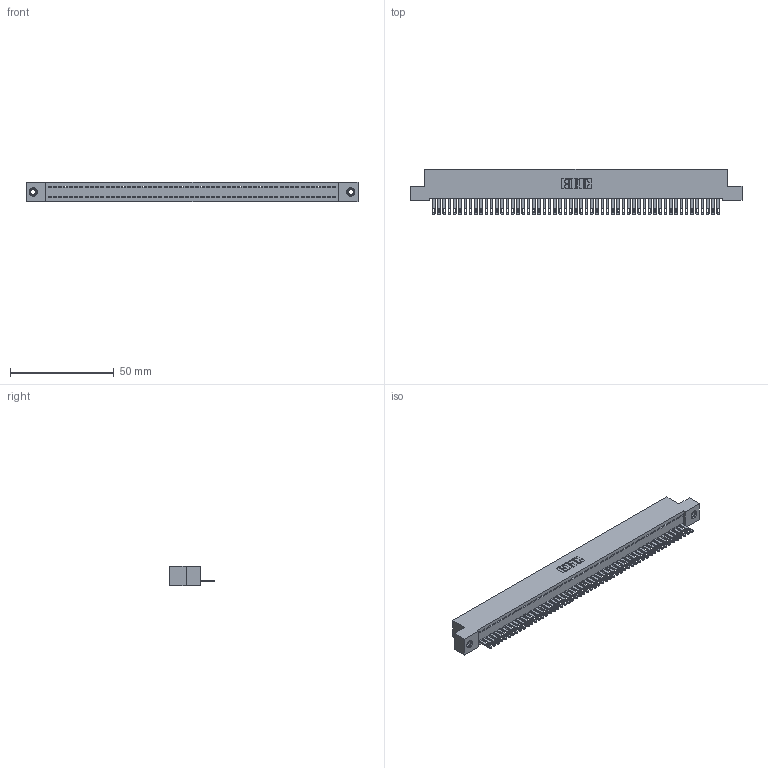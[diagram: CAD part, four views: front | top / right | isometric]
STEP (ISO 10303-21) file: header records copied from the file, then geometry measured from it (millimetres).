
FILE_DESCRIPTION (( 'STEP AP203' ), '1' );
FILE_NAME ('892-055-500-107.STEP', '2020-09-21T18:33:28', ( '' ), ( '' ), 'SwSTEP 2.0', 'SolidWorks 2020', '' );
FILE_SCHEMA (( 'CONFIG_CONTROL_DESIGN' ));
Length unit declared in the file: inch
Products named in the file (4): 345-292-001_345-293-100; 345-250-001_345-250-005-103; 892-055-500-107; 842 Part_TI
Assembly tree (58 placements, depth 2):
  892-055-500-107
    842 Part_TI
    345-292-001_345-293-100  x55
    345-250-001_345-250-005-103  x2
Bounding box: 160.02 x 21.85 x 9.4 mm (x, y, z)
Volume: 14099.8 mm3; surface area: 21088.1 mm2
Topology: 58 solids, 58 shells, 3140 faces, 9675 edges, 6442 vertices
Faces by surface type: plane 2078, cylinder 1046, cone 12, torus 4
Entity records: 32926 total; most frequent: CARTESIAN_POINT 5658, ORIENTED_EDGE 5642, DIRECTION 4781, EDGE_CURVE 2821, LINE 2669, VECTOR 2669, VERTEX_POINT 1876, AXIS2_PLACEMENT_3D 1056
